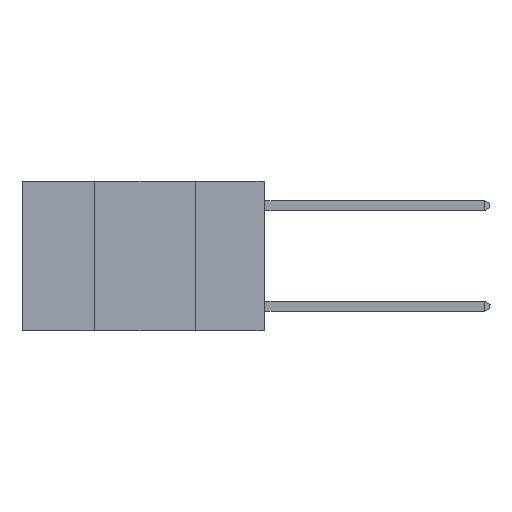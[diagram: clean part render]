
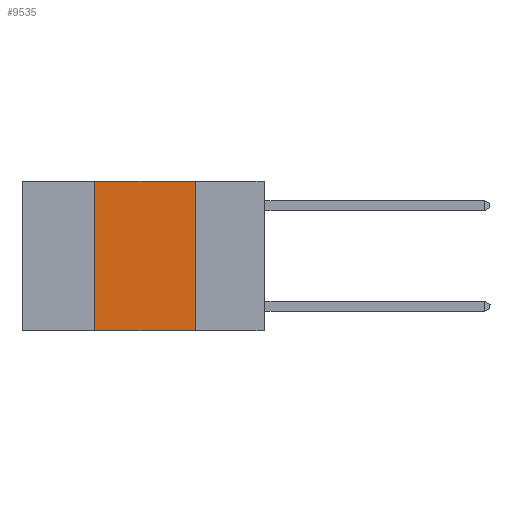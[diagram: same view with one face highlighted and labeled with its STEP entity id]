
A CAD part, left-side view. The second image highlights one B-rep face of the part: STEP entity #9535.
In plain terms, the highlighted planar face has unit normal (-1, 0, 0).
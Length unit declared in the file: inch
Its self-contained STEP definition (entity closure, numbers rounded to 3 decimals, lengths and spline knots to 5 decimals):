
#327 = CARTESIAN_POINT ( 'NONE',  ( 0., 0.6, 0. ) ) ;
#398 = AXIS2_PLACEMENT_3D ( 'NONE', #13908, #15341, #6704 ) ;
#908 = ORIENTED_EDGE ( 'NONE', *, *, #3019, .T. ) ;
#3019 = EDGE_CURVE ( 'NONE', #17126, #6677, #6250, .T. ) ;
#3058 = VECTOR ( 'NONE', #9648, 39.37008 ) ;
#3449 = EDGE_CURVE ( 'NONE', #17126, #5558, #17830, .T. ) ;
#4552 = EDGE_CURVE ( 'NONE', #9772, #6677, #10103, .T. ) ;
#5373 = ORIENTED_EDGE ( 'NONE', *, *, #8312, .F. ) ;
#5484 = CARTESIAN_POINT ( 'NONE',  ( 0., 0.6, -0.37 ) ) ;
#5558 = VERTEX_POINT ( 'NONE', #8184 ) ;
#6250 = LINE ( 'NONE', #5484, #12576 ) ;
#6589 = ORIENTED_EDGE ( 'NONE', *, *, #4552, .F. ) ;
#6677 = VERTEX_POINT ( 'NONE', #13227 ) ;
#6704 = DIRECTION ( 'NONE',  ( 0., 0., -1. ) ) ;
#7247 = FACE_OUTER_BOUND ( 'NONE', #16863, .T. ) ;
#8184 = CARTESIAN_POINT ( 'NONE',  ( 0., 0.42, 0. ) ) ;
#8312 = EDGE_CURVE ( 'NONE', #5558, #9772, #9851, .T. ) ;
#9012 = CARTESIAN_POINT ( 'NONE',  ( 0., 0.42, -0.37 ) ) ;
#9535 = ADVANCED_FACE ( 'NONE', ( #7247 ), #12450, .F. ) ;
#9648 = DIRECTION ( 'NONE',  ( 0., 0., -1. ) ) ;
#9772 = VERTEX_POINT ( 'NONE', #17358 ) ;
#9851 = LINE ( 'NONE', #327, #13157 ) ;
#10103 = LINE ( 'NONE', #18052, #3058 ) ;
#12450 = PLANE ( 'NONE',  #398 ) ;
#12576 = VECTOR ( 'NONE', #15748, 39.37008 ) ;
#12894 = DIRECTION ( 'NONE',  ( 0., 0., 1. ) ) ;
#13157 = VECTOR ( 'NONE', #13643, 39.37008 ) ;
#13227 = CARTESIAN_POINT ( 'NONE',  ( 0., 0.17, -0.37 ) ) ;
#13404 = ORIENTED_EDGE ( 'NONE', *, *, #3449, .F. ) ;
#13643 = DIRECTION ( 'NONE',  ( 0., -1., 0. ) ) ;
#13908 = CARTESIAN_POINT ( 'NONE',  ( 0., 0.6, 0. ) ) ;
#15341 = DIRECTION ( 'NONE',  ( 1., 0., 0. ) ) ;
#15748 = DIRECTION ( 'NONE',  ( 0., -1., 0. ) ) ;
#16863 = EDGE_LOOP ( 'NONE', ( #6589, #5373, #13404, #908 ) ) ;
#17077 = CARTESIAN_POINT ( 'NONE',  ( 0., 0.42, 0. ) ) ;
#17126 = VERTEX_POINT ( 'NONE', #9012 ) ;
#17358 = CARTESIAN_POINT ( 'NONE',  ( 0., 0.17, 0. ) ) ;
#17389 = VECTOR ( 'NONE', #12894, 39.37008 ) ;
#17830 = LINE ( 'NONE', #17077, #17389 ) ;
#18052 = CARTESIAN_POINT ( 'NONE',  ( 0., 0.17, 0. ) ) ;
